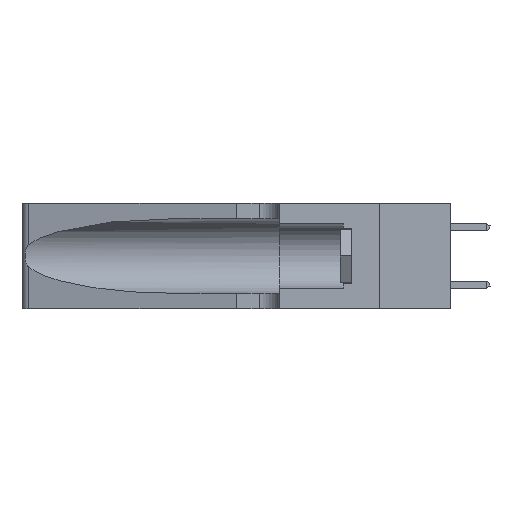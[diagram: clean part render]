
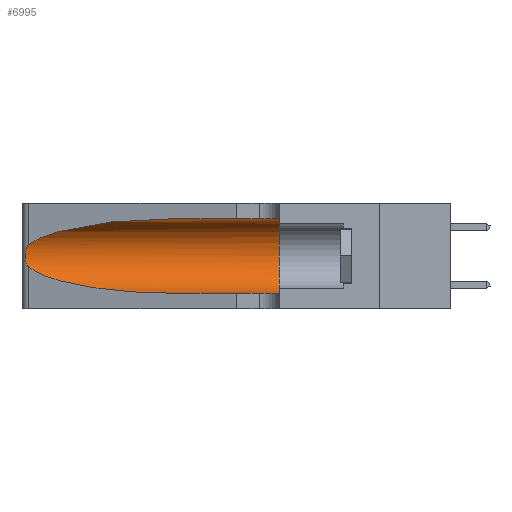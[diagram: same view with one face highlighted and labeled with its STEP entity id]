
A CAD part, left-side view. The second image highlights one B-rep face of the part: STEP entity #6995.
In plain terms, the highlighted cylindrical face has radius 3.308 mm (diameter 6.617 mm), a partial arc.
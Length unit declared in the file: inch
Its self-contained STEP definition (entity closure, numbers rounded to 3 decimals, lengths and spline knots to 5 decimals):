
#228 = CARTESIAN_POINT ( 'NONE',  ( 0.2373, 1.15595, 0.28018 ) ) ;
#734 = CARTESIAN_POINT ( 'NONE',  ( 0.25487, 1.22718, 0.14631 ) ) ;
#771 =( BOUNDED_CURVE ( )  B_SPLINE_CURVE ( 3, ( #18225, #3210, #228, #12329 ),
 .UNSPECIFIED., .F., .F. ) 
 B_SPLINE_CURVE_WITH_KNOTS ( ( 4, 4 ),
 ( 1.5708, 2.84003 ),
 .UNSPECIFIED. ) 
 CURVE ( )  GEOMETRIC_REPRESENTATION_ITEM ( )  RATIONAL_B_SPLINE_CURVE ( ( 1., 0.87, 0.87, 1. ) ) 
 REPRESENTATION_ITEM ( '' )  );
#863 = EDGE_CURVE ( 'NONE', #9922, #7782, #13611, .T. ) ;
#913 = EDGE_CURVE ( 'NONE', #13150, #3472, #6580, .T. ) ;
#936 = CARTESIAN_POINT ( 'NONE',  ( 0.25639, 1.23186, 0.15144 ) ) ;
#3210 = CARTESIAN_POINT ( 'NONE',  ( 0.18966, 0.96281, 0.31525 ) ) ;
#3472 = VERTEX_POINT ( 'NONE', #13434 ) ;
#3786 = AXIS2_PLACEMENT_3D ( 'NONE', #13564, #19510, #13505 ) ;
#3944 = VERTEX_POINT ( 'NONE', #18502 ) ;
#4125 = DIRECTION ( 'NONE',  ( 0., -1., 0. ) ) ;
#4366 = CARTESIAN_POINT ( 'NONE',  ( 0.25487, 1.22718, 0.22369 ) ) ;
#4645 = EDGE_CURVE ( 'NONE', #6786, #3944, #771, .T. ) ;
#5528 = CARTESIAN_POINT ( 'NONE',  ( 0.26018, 1.23835, 0.19895 ) ) ;
#5617 = VECTOR ( 'NONE', #4125, 39.37008 ) ;
#5712 = CARTESIAN_POINT ( 'NONE',  ( 0.25789, 1.23486, 0.15765 ) ) ;
#6280 = CARTESIAN_POINT ( 'NONE',  ( 0.26017, 1.23833, 0.17102 ) ) ;
#6354 = EDGE_CURVE ( 'NONE', #7782, #3472, #13157, .T. ) ;
#6474 = ORIENTED_EDGE ( 'NONE', *, *, #11164, .T. ) ;
#6490 = CARTESIAN_POINT ( 'NONE',  ( 0.25787, 1.23484, 0.2124 ) ) ;
#6580 = CIRCLE ( 'NONE', #15598, 0.13025 ) ;
#6786 = VERTEX_POINT ( 'NONE', #11929 ) ;
#6908 = CARTESIAN_POINT ( 'NONE',  ( 0.1305, 0.72297, 0.05475 ) ) ;
#6995 = ADVANCED_FACE ( 'NONE', ( #16678 ), #17836, .F. ) ;
#7053 = DIRECTION ( 'NONE',  ( 0., 1., 0. ) ) ;
#7646 = CARTESIAN_POINT ( 'NONE',  ( 0.26075, 1.23896, 0.178 ) ) ;
#7782 = VERTEX_POINT ( 'NONE', #11041 ) ;
#7839 = LINE ( 'NONE', #8532, #17006 ) ;
#8532 = CARTESIAN_POINT ( 'NONE',  ( 0.1305, 1.61858, 0.31525 ) ) ;
#8630 = CARTESIAN_POINT ( 'NONE',  ( 0.25487, 1.22718, 0.14631 ) ) ;
#8702 = DIRECTION ( 'NONE',  ( 0., 0., 1. ) ) ;
#8930 = ORIENTED_EDGE ( 'NONE', *, *, #10312, .F. ) ;
#9707 = CARTESIAN_POINT ( 'NONE',  ( 0.25555, 1.22994, 0.2215 ) ) ;
#9922 = VERTEX_POINT ( 'NONE', #13216 ) ;
#10217 = CARTESIAN_POINT ( 'NONE',  ( 0.1305, 1.61858, 0.05475 ) ) ;
#10312 = EDGE_CURVE ( 'NONE', #6786, #13150, #7839, .T. ) ;
#10441 = CARTESIAN_POINT ( 'NONE',  ( 0.26075, 1.23896, 0.19203 ) ) ;
#11041 = CARTESIAN_POINT ( 'NONE',  ( 0.1305, 0.72297, 0.05475 ) ) ;
#11164 = EDGE_CURVE ( 'NONE', #3944, #9922, #12768, .T. ) ;
#11929 = CARTESIAN_POINT ( 'NONE',  ( 0.1305, 0.72297, 0.31525 ) ) ;
#12204 = ORIENTED_EDGE ( 'NONE', *, *, #913, .F. ) ;
#12329 = CARTESIAN_POINT ( 'NONE',  ( 0.25487, 1.22718, 0.22369 ) ) ;
#12768 = B_SPLINE_CURVE_WITH_KNOTS ( 'NONE', 3,
 ( #4366, #9707, #15738, #6490, #15936, #5528, #10441, #7646, #6280, #17605, #5712, #936, #17538, #8630 ),
 .UNSPECIFIED., .F., .F.,
 ( 4, 2, 2, 2, 2, 2, 4 ),
 ( 0., 0.00027, 0.00053, 0.00107, 0.0016, 0.00187, 0.00214 ),
 .UNSPECIFIED. ) ;
#13150 = VERTEX_POINT ( 'NONE', #17351 ) ;
#13157 = LINE ( 'NONE', #10217, #5617 ) ;
#13216 = CARTESIAN_POINT ( 'NONE',  ( 0.25487, 1.22718, 0.14631 ) ) ;
#13253 = DIRECTION ( 'NONE',  ( 0., -1., 0. ) ) ;
#13434 = CARTESIAN_POINT ( 'NONE',  ( 0.1305, 0.35, 0.05475 ) ) ;
#13464 = ORIENTED_EDGE ( 'NONE', *, *, #863, .T. ) ;
#13505 = DIRECTION ( 'NONE',  ( 0., 0., -1. ) ) ;
#13564 = CARTESIAN_POINT ( 'NONE',  ( 0.1305, 1.61858, 0.185 ) ) ;
#13611 =( BOUNDED_CURVE ( )  B_SPLINE_CURVE ( 3, ( #734, #17471, #15908, #6908 ),
 .UNSPECIFIED., .F., .F. ) 
 B_SPLINE_CURVE_WITH_KNOTS ( ( 4, 4 ),
 ( 3.44316, 4.71239 ),
 .UNSPECIFIED. ) 
 CURVE ( )  GEOMETRIC_REPRESENTATION_ITEM ( )  RATIONAL_B_SPLINE_CURVE ( ( 1., 0.87, 0.87, 1. ) ) 
 REPRESENTATION_ITEM ( '' )  );
#15140 = ORIENTED_EDGE ( 'NONE', *, *, #4645, .T. ) ;
#15598 = AXIS2_PLACEMENT_3D ( 'NONE', #16304, #7053, #8702 ) ;
#15738 = CARTESIAN_POINT ( 'NONE',  ( 0.25639, 1.23184, 0.21858 ) ) ;
#15908 = CARTESIAN_POINT ( 'NONE',  ( 0.18966, 0.96281, 0.05475 ) ) ;
#15936 = CARTESIAN_POINT ( 'NONE',  ( 0.25854, 1.2359, 0.20912 ) ) ;
#16304 = CARTESIAN_POINT ( 'NONE',  ( 0.1305, 0.35, 0.185 ) ) ;
#16678 = FACE_OUTER_BOUND ( 'NONE', #17609, .T. ) ;
#16798 = ORIENTED_EDGE ( 'NONE', *, *, #6354, .T. ) ;
#17006 = VECTOR ( 'NONE', #13253, 39.37008 ) ;
#17351 = CARTESIAN_POINT ( 'NONE',  ( 0.1305, 0.35, 0.31525 ) ) ;
#17471 = CARTESIAN_POINT ( 'NONE',  ( 0.2373, 1.15595, 0.08982 ) ) ;
#17538 = CARTESIAN_POINT ( 'NONE',  ( 0.25555, 1.22993, 0.14849 ) ) ;
#17605 = CARTESIAN_POINT ( 'NONE',  ( 0.25856, 1.23593, 0.16098 ) ) ;
#17609 = EDGE_LOOP ( 'NONE', ( #15140, #6474, #13464, #16798, #12204, #8930 ) ) ;
#17836 = CYLINDRICAL_SURFACE ( 'NONE', #3786, 0.13025 ) ;
#18225 = CARTESIAN_POINT ( 'NONE',  ( 0.1305, 0.72297, 0.31525 ) ) ;
#18502 = CARTESIAN_POINT ( 'NONE',  ( 0.25487, 1.22718, 0.22369 ) ) ;
#19510 = DIRECTION ( 'NONE',  ( 0., -1., 0. ) ) ;
